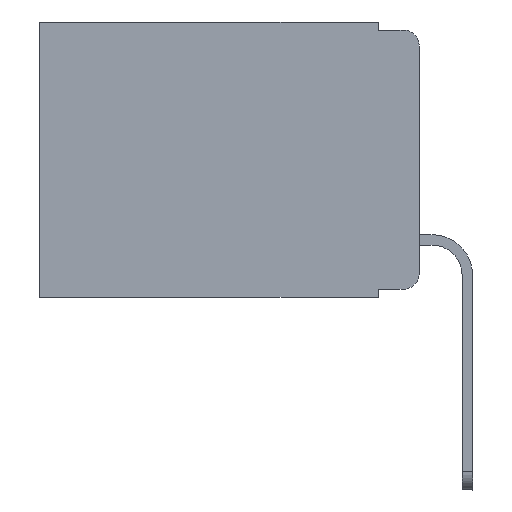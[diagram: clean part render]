
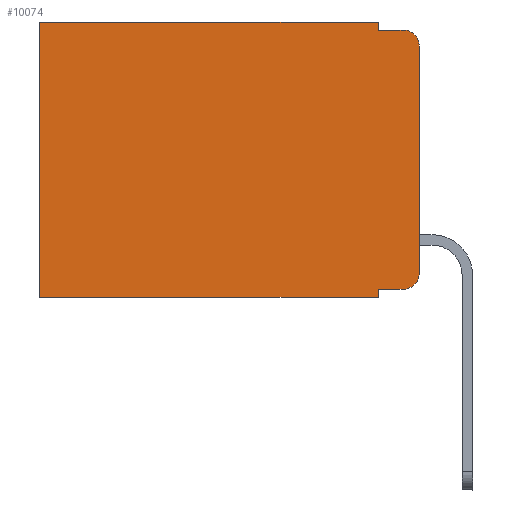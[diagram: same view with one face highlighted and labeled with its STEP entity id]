
A CAD part, left-side view. The second image highlights one B-rep face of the part: STEP entity #10074.
In plain terms, the highlighted planar face has unit normal (-1, 0, 0).
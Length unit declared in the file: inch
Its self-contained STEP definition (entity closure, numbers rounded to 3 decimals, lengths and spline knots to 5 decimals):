
#56 = DIRECTION ( 'NONE',  ( 0., 0., -1. ) ) ;
#113 = ORIENTED_EDGE ( 'NONE', *, *, #8088, .T. ) ;
#242 = CARTESIAN_POINT ( 'NONE',  ( 0.298, 0.051, 0. ) ) ;
#419 = EDGE_CURVE ( 'NONE', #11989, #4213, #12959, .T. ) ;
#878 = VECTOR ( 'NONE', #9811, 39.37008 ) ;
#974 = VERTEX_POINT ( 'NONE', #15487 ) ;
#1077 = EDGE_CURVE ( 'NONE', #11117, #2993, #11809, .T. ) ;
#1716 = CARTESIAN_POINT ( 'NONE',  ( 0.298, 0.051, -0.01 ) ) ;
#1965 = VECTOR ( 'NONE', #18734, 39.37008 ) ;
#2680 = DIRECTION ( 'NONE',  ( -1., 0., 0. ) ) ;
#2704 = VERTEX_POINT ( 'NONE', #12640 ) ;
#2752 = AXIS2_PLACEMENT_3D ( 'NONE', #18687, #2680, #5575 ) ;
#2993 = VERTEX_POINT ( 'NONE', #18395 ) ;
#3134 = FACE_OUTER_BOUND ( 'NONE', #3949, .T. ) ;
#3662 = LINE ( 'NONE', #12715, #878 ) ;
#3775 = ORIENTED_EDGE ( 'NONE', *, *, #8733, .F. ) ;
#3814 = VERTEX_POINT ( 'NONE', #6754 ) ;
#3949 = EDGE_LOOP ( 'NONE', ( #3775, #7173, #6657, #5694, #8672, #8048, #5069, #13112, #11147, #113 ) ) ;
#4213 = VERTEX_POINT ( 'NONE', #18114 ) ;
#4447 = EDGE_CURVE ( 'NONE', #5986, #4213, #5440, .T. ) ;
#4781 = VECTOR ( 'NONE', #6709, 39.37008 ) ;
#4887 = VECTOR ( 'NONE', #17605, 39.37008 ) ;
#5069 = ORIENTED_EDGE ( 'NONE', *, *, #9893, .F. ) ;
#5440 = CIRCLE ( 'NONE', #11922, 0.02 ) ;
#5556 = CARTESIAN_POINT ( 'NONE',  ( 0.298, 0., -0.343 ) ) ;
#5575 = DIRECTION ( 'NONE',  ( 0., 0., -1. ) ) ;
#5694 = ORIENTED_EDGE ( 'NONE', *, *, #9772, .F. ) ;
#5926 = LINE ( 'NONE', #6123, #18871 ) ;
#5986 = VERTEX_POINT ( 'NONE', #9973 ) ;
#6048 = DIRECTION ( 'NONE',  ( -1., 0., 0. ) ) ;
#6123 = CARTESIAN_POINT ( 'NONE',  ( 0.298, 0., 0. ) ) ;
#6657 = ORIENTED_EDGE ( 'NONE', *, *, #419, .F. ) ;
#6709 = DIRECTION ( 'NONE',  ( 0., 0., -1. ) ) ;
#6754 = CARTESIAN_POINT ( 'NONE',  ( 0.298, 0.051, -0.333 ) ) ;
#7173 = ORIENTED_EDGE ( 'NONE', *, *, #4447, .T. ) ;
#7567 = PLANE ( 'NONE',  #18892 ) ;
#8048 = ORIENTED_EDGE ( 'NONE', *, *, #1077, .T. ) ;
#8088 = EDGE_CURVE ( 'NONE', #15542, #2704, #13810, .T. ) ;
#8090 = EDGE_CURVE ( 'NONE', #3814, #974, #18782, .T. ) ;
#8672 = ORIENTED_EDGE ( 'NONE', *, *, #13391, .T. ) ;
#8733 = EDGE_CURVE ( 'NONE', #5986, #2704, #5926, .T. ) ;
#8744 = DIRECTION ( 'NONE',  ( 0., 0., -1. ) ) ;
#9690 = CARTESIAN_POINT ( 'NONE',  ( 0.298, 0.051, -0.333 ) ) ;
#9772 = EDGE_CURVE ( 'NONE', #11025, #11989, #16766, .T. ) ;
#9811 = DIRECTION ( 'NONE',  ( 0., 1., 0. ) ) ;
#9893 = EDGE_CURVE ( 'NONE', #974, #2993, #18763, .T. ) ;
#9973 = CARTESIAN_POINT ( 'NONE',  ( 0.298, 0., -0.03 ) ) ;
#10027 = VECTOR ( 'NONE', #11723, 39.37008 ) ;
#10074 = ADVANCED_FACE ( 'NONE', ( #3134 ), #7567, .F. ) ;
#10473 = CARTESIAN_POINT ( 'NONE',  ( 0.298, 0.02, -0.03 ) ) ;
#11025 = VERTEX_POINT ( 'NONE', #242 ) ;
#11117 = VERTEX_POINT ( 'NONE', #14672 ) ;
#11119 = CARTESIAN_POINT ( 'NONE',  ( 0.298, 0., 0. ) ) ;
#11147 = ORIENTED_EDGE ( 'NONE', *, *, #15872, .T. ) ;
#11452 = DIRECTION ( 'NONE',  ( 0., 0., -1. ) ) ;
#11723 = DIRECTION ( 'NONE',  ( 0., 1., 0. ) ) ;
#11809 = LINE ( 'NONE', #13340, #4887 ) ;
#11922 = AXIS2_PLACEMENT_3D ( 'NONE', #10473, #6048, #8744 ) ;
#11989 = VERTEX_POINT ( 'NONE', #1716 ) ;
#12640 = CARTESIAN_POINT ( 'NONE',  ( 0.298, 0., -0.313 ) ) ;
#12715 = CARTESIAN_POINT ( 'NONE',  ( 0.298, 0., 0. ) ) ;
#12959 = LINE ( 'NONE', #15694, #1965 ) ;
#13112 = ORIENTED_EDGE ( 'NONE', *, *, #8090, .F. ) ;
#13340 = CARTESIAN_POINT ( 'NONE',  ( 0.298, 0.473, 0. ) ) ;
#13391 = EDGE_CURVE ( 'NONE', #11025, #11117, #3662, .T. ) ;
#13510 = VECTOR ( 'NONE', #11452, 39.37008 ) ;
#13654 = DIRECTION ( 'NONE',  ( 0., -1., 0. ) ) ;
#13810 = CIRCLE ( 'NONE', #2752, 0.02 ) ;
#14005 = CARTESIAN_POINT ( 'NONE',  ( 0.298, 0.051, 0. ) ) ;
#14672 = CARTESIAN_POINT ( 'NONE',  ( 0.298, 0.473, 0. ) ) ;
#15487 = CARTESIAN_POINT ( 'NONE',  ( 0.298, 0.051, -0.343 ) ) ;
#15542 = VERTEX_POINT ( 'NONE', #15662 ) ;
#15662 = CARTESIAN_POINT ( 'NONE',  ( 0.298, 0.02, -0.333 ) ) ;
#15694 = CARTESIAN_POINT ( 'NONE',  ( 0.298, 0.051, -0.01 ) ) ;
#15742 = CARTESIAN_POINT ( 'NONE',  ( 0.298, 0.051, 0. ) ) ;
#15872 = EDGE_CURVE ( 'NONE', #3814, #15542, #16595, .T. ) ;
#16595 = LINE ( 'NONE', #9690, #17250 ) ;
#16766 = LINE ( 'NONE', #14005, #4781 ) ;
#16836 = DIRECTION ( 'NONE',  ( 0., 0., -1. ) ) ;
#17250 = VECTOR ( 'NONE', #13654, 39.37008 ) ;
#17605 = DIRECTION ( 'NONE',  ( 0., 0., -1. ) ) ;
#18114 = CARTESIAN_POINT ( 'NONE',  ( 0.298, 0.02, -0.01 ) ) ;
#18163 = DIRECTION ( 'NONE',  ( 1., 0., 0. ) ) ;
#18395 = CARTESIAN_POINT ( 'NONE',  ( 0.298, 0.473, -0.343 ) ) ;
#18687 = CARTESIAN_POINT ( 'NONE',  ( 0.298, 0.02, -0.313 ) ) ;
#18734 = DIRECTION ( 'NONE',  ( 0., -1., 0. ) ) ;
#18763 = LINE ( 'NONE', #5556, #10027 ) ;
#18782 = LINE ( 'NONE', #15742, #13510 ) ;
#18871 = VECTOR ( 'NONE', #56, 39.37008 ) ;
#18892 = AXIS2_PLACEMENT_3D ( 'NONE', #11119, #18163, #16836 ) ;
